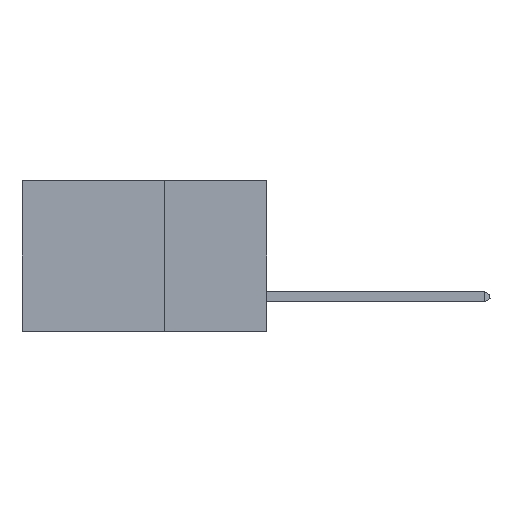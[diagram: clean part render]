
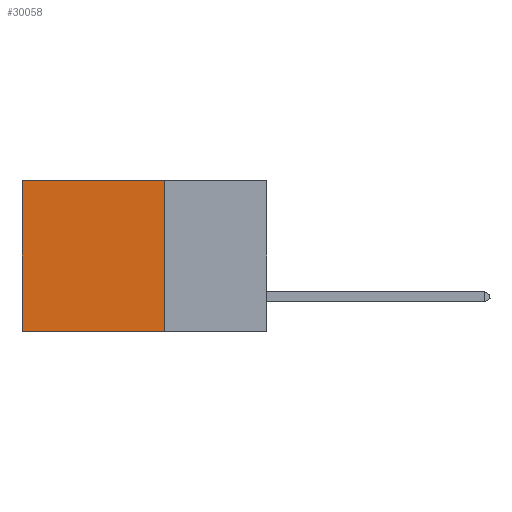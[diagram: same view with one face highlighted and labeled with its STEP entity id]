
A CAD part, left-side view. The second image highlights one B-rep face of the part: STEP entity #30058.
In plain terms, the highlighted planar face has unit normal (-1, 0, 0).
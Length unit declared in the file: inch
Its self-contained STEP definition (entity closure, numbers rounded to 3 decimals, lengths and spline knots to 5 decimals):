
#358 = CARTESIAN_POINT ( 'NONE',  ( 0.2875, 0.25, -0.37 ) ) ;
#4164 = VECTOR ( 'NONE', #19514, 39.37008 ) ;
#5012 = CARTESIAN_POINT ( 'NONE',  ( 0.2875, 0.25, 0. ) ) ;
#5467 = DIRECTION ( 'NONE',  ( 0., 0., -1. ) ) ;
#6674 = DIRECTION ( 'NONE',  ( 1., 0., 0. ) ) ;
#6802 = DIRECTION ( 'NONE',  ( 0., 0., -1. ) ) ;
#7049 = PLANE ( 'NONE',  #25775 ) ;
#7752 = DIRECTION ( 'NONE',  ( 0., 0., -1. ) ) ;
#10324 = CARTESIAN_POINT ( 'NONE',  ( 0.2875, 0.25, 0. ) ) ;
#12483 = EDGE_CURVE ( 'NONE', #16243, #32844, #37013, .T. ) ;
#13010 = EDGE_CURVE ( 'NONE', #32844, #27925, #24545, .T. ) ;
#14190 = CARTESIAN_POINT ( 'NONE',  ( 0.2875, 0.6, 0. ) ) ;
#16138 = DIRECTION ( 'NONE',  ( 0., 1., 0. ) ) ;
#16243 = VERTEX_POINT ( 'NONE', #37611 ) ;
#16636 = VECTOR ( 'NONE', #16138, 39.37008 ) ;
#16639 = CARTESIAN_POINT ( 'NONE',  ( 0.2875, 0.25, -0.37 ) ) ;
#19254 = CARTESIAN_POINT ( 'NONE',  ( 0.2875, 0.6, -0.37 ) ) ;
#19514 = DIRECTION ( 'NONE',  ( 0., 1., 0. ) ) ;
#20647 = CARTESIAN_POINT ( 'NONE',  ( 0.2875, 0.6, 0. ) ) ;
#21357 = CARTESIAN_POINT ( 'NONE',  ( 0.2875, 0.25, 0. ) ) ;
#24053 = EDGE_CURVE ( 'NONE', #16243, #27655, #35645, .T. ) ;
#24545 = LINE ( 'NONE', #16639, #16636 ) ;
#25388 = EDGE_LOOP ( 'NONE', ( #26971, #30660, #31778, #26464 ) ) ;
#25775 = AXIS2_PLACEMENT_3D ( 'NONE', #21357, #6674, #6802 ) ;
#26464 = ORIENTED_EDGE ( 'NONE', *, *, #24053, .T. ) ;
#26971 = ORIENTED_EDGE ( 'NONE', *, *, #37824, .T. ) ;
#27655 = VERTEX_POINT ( 'NONE', #14190 ) ;
#27925 = VERTEX_POINT ( 'NONE', #19254 ) ;
#29142 = VECTOR ( 'NONE', #7752, 39.37008 ) ;
#29968 = FACE_OUTER_BOUND ( 'NONE', #25388, .T. ) ;
#30058 = ADVANCED_FACE ( 'NONE', ( #29968 ), #7049, .F. ) ;
#30660 = ORIENTED_EDGE ( 'NONE', *, *, #13010, .F. ) ;
#31778 = ORIENTED_EDGE ( 'NONE', *, *, #12483, .F. ) ;
#32844 = VERTEX_POINT ( 'NONE', #358 ) ;
#33052 = VECTOR ( 'NONE', #5467, 39.37008 ) ;
#35645 = LINE ( 'NONE', #10324, #4164 ) ;
#37013 = LINE ( 'NONE', #5012, #29142 ) ;
#37611 = CARTESIAN_POINT ( 'NONE',  ( 0.2875, 0.25, 0. ) ) ;
#37824 = EDGE_CURVE ( 'NONE', #27655, #27925, #38149, .T. ) ;
#38149 = LINE ( 'NONE', #20647, #33052 ) ;
